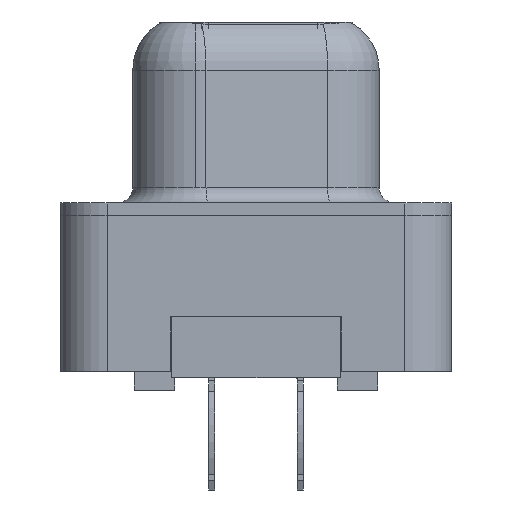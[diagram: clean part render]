
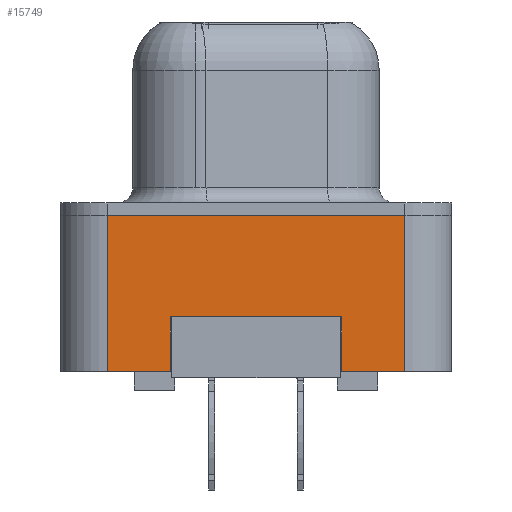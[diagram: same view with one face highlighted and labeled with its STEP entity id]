
A CAD part, left-side view. The second image highlights one B-rep face of the part: STEP entity #15749.
In plain terms, the highlighted planar face has unit normal (-1, 0, 0).
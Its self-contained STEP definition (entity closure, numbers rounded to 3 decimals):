
#19 = VERTEX_POINT ( 'NONE', #9708 ) ;
#203 = DIRECTION ( 'NONE',  ( 0., 0., 1. ) ) ;
#410 = DIRECTION ( 'NONE',  ( 0., 0., -1. ) ) ;
#2005 = VERTEX_POINT ( 'NONE', #13542 ) ;
#2590 = VERTEX_POINT ( 'NONE', #9658 ) ;
#3083 = VECTOR ( 'NONE', #6466, 1000. ) ;
#3212 = EDGE_CURVE ( 'NONE', #11833, #19, #20085, .T. ) ;
#4068 = ORIENTED_EDGE ( 'NONE', *, *, #16184, .T. ) ;
#4280 = EDGE_CURVE ( 'NONE', #2005, #2590, #16799, .T. ) ;
#4455 = DIRECTION ( 'NONE',  ( 0., -1., 0. ) ) ;
#4665 = EDGE_CURVE ( 'NONE', #10159, #19, #8056, .T. ) ;
#5027 = DIRECTION ( 'NONE',  ( 0., 0., 1. ) ) ;
#5321 = DIRECTION ( 'NONE',  ( 0., -1., 0. ) ) ;
#6234 = CARTESIAN_POINT ( 'NONE',  ( -2.995, -4.775, -5. ) ) ;
#6376 = DIRECTION ( 'NONE',  ( 0., -1., 0. ) ) ;
#6466 = DIRECTION ( 'NONE',  ( 0., 0., -1. ) ) ;
#6719 = CARTESIAN_POINT ( 'NONE',  ( -2.995, 4.775, -5. ) ) ;
#6892 = CARTESIAN_POINT ( 'NONE',  ( -2.995, -2.75, -3.25 ) ) ;
#6895 = LINE ( 'NONE', #9002, #7282 ) ;
#6993 = LINE ( 'NONE', #20622, #10561 ) ;
#7282 = VECTOR ( 'NONE', #410, 1000. ) ;
#7449 = ORIENTED_EDGE ( 'NONE', *, *, #9976, .F. ) ;
#7802 = CARTESIAN_POINT ( 'NONE',  ( -2.995, -4.775, 0. ) ) ;
#8052 = LINE ( 'NONE', #14857, #8508 ) ;
#8056 = LINE ( 'NONE', #13179, #13019 ) ;
#8307 = CARTESIAN_POINT ( 'NONE',  ( -2.995, 2.75, -3.25 ) ) ;
#8508 = VECTOR ( 'NONE', #6376, 1000. ) ;
#8726 = CARTESIAN_POINT ( 'NONE',  ( -2.995, 4.775, 0. ) ) ;
#9002 = CARTESIAN_POINT ( 'NONE',  ( -2.995, 2.75, -3.25 ) ) ;
#9243 = LINE ( 'NONE', #9358, #17286 ) ;
#9358 = CARTESIAN_POINT ( 'NONE',  ( -2.995, 4.775, -5. ) ) ;
#9577 = ORIENTED_EDGE ( 'NONE', *, *, #10446, .T. ) ;
#9658 = CARTESIAN_POINT ( 'NONE',  ( -2.995, 2.75, -3.25 ) ) ;
#9708 = CARTESIAN_POINT ( 'NONE',  ( -2.995, -4.775, 0. ) ) ;
#9922 = ORIENTED_EDGE ( 'NONE', *, *, #4280, .F. ) ;
#9976 = EDGE_CURVE ( 'NONE', #16598, #11833, #9243, .T. ) ;
#10159 = VERTEX_POINT ( 'NONE', #6234 ) ;
#10230 = VERTEX_POINT ( 'NONE', #11459 ) ;
#10446 = EDGE_CURVE ( 'NONE', #16598, #21808, #6993, .T. ) ;
#10561 = VECTOR ( 'NONE', #5321, 1000. ) ;
#11459 = CARTESIAN_POINT ( 'NONE',  ( -2.995, -2.75, -5. ) ) ;
#11833 = VERTEX_POINT ( 'NONE', #8726 ) ;
#12549 = ORIENTED_EDGE ( 'NONE', *, *, #4665, .T. ) ;
#12577 = FACE_OUTER_BOUND ( 'NONE', #14561, .T. ) ;
#12595 = EDGE_CURVE ( 'NONE', #2590, #21808, #6895, .T. ) ;
#13019 = VECTOR ( 'NONE', #5027, 1000. ) ;
#13179 = CARTESIAN_POINT ( 'NONE',  ( -2.995, -4.775, -5. ) ) ;
#13353 = VECTOR ( 'NONE', #15113, 1000. ) ;
#13542 = CARTESIAN_POINT ( 'NONE',  ( -2.995, -2.75, -3.25 ) ) ;
#13928 = VECTOR ( 'NONE', #4455, 1000. ) ;
#13935 = DIRECTION ( 'NONE',  ( -1., 0., 0. ) ) ;
#14561 = EDGE_LOOP ( 'NONE', ( #4068, #16666, #12549, #19736, #7449, #9577, #14569, #9922 ) ) ;
#14569 = ORIENTED_EDGE ( 'NONE', *, *, #12595, .F. ) ;
#14837 = AXIS2_PLACEMENT_3D ( 'NONE', #17191, #13935, #203 ) ;
#14857 = CARTESIAN_POINT ( 'NONE',  ( -2.995, -4.775, -5. ) ) ;
#14945 = LINE ( 'NONE', #6892, #3083 ) ;
#15113 = DIRECTION ( 'NONE',  ( 0., 1., 0. ) ) ;
#15749 = ADVANCED_FACE ( 'NONE', ( #12577 ), #19404, .T. ) ;
#16064 = DIRECTION ( 'NONE',  ( 0., 0., 1. ) ) ;
#16184 = EDGE_CURVE ( 'NONE', #2005, #10230, #14945, .T. ) ;
#16598 = VERTEX_POINT ( 'NONE', #6719 ) ;
#16666 = ORIENTED_EDGE ( 'NONE', *, *, #18995, .T. ) ;
#16799 = LINE ( 'NONE', #8307, #13353 ) ;
#17191 = CARTESIAN_POINT ( 'NONE',  ( -2.995, -4.775, -5. ) ) ;
#17286 = VECTOR ( 'NONE', #16064, 1000. ) ;
#18995 = EDGE_CURVE ( 'NONE', #10230, #10159, #8052, .T. ) ;
#19404 = PLANE ( 'NONE',  #14837 ) ;
#19736 = ORIENTED_EDGE ( 'NONE', *, *, #3212, .F. ) ;
#20085 = LINE ( 'NONE', #7802, #13928 ) ;
#20622 = CARTESIAN_POINT ( 'NONE',  ( -2.995, -4.775, -5. ) ) ;
#21212 = CARTESIAN_POINT ( 'NONE',  ( -2.995, 2.75, -5. ) ) ;
#21808 = VERTEX_POINT ( 'NONE', #21212 ) ;
